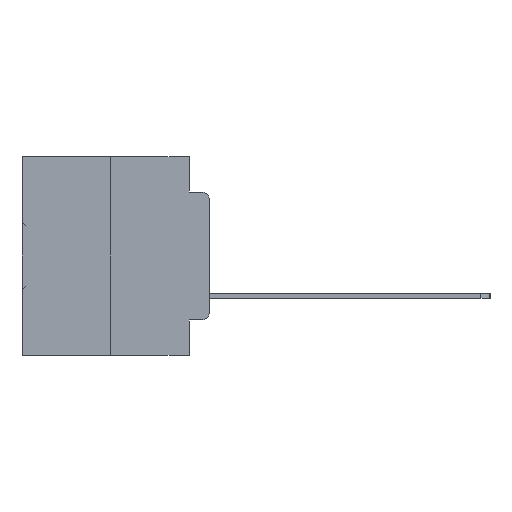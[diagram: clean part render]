
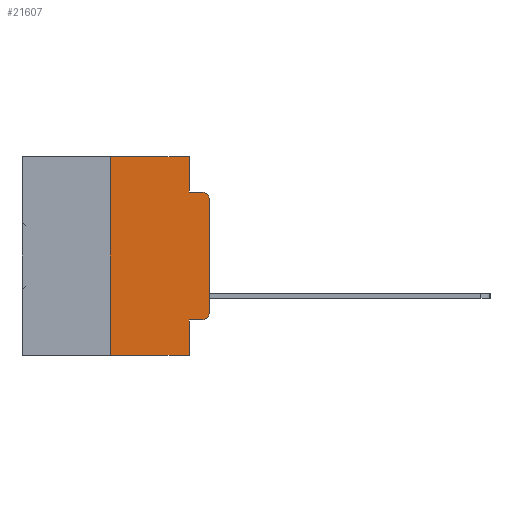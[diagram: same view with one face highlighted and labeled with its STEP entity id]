
A CAD part, left-side view. The second image highlights one B-rep face of the part: STEP entity #21607.
In plain terms, the highlighted planar face has unit normal (-1, 0, 0).
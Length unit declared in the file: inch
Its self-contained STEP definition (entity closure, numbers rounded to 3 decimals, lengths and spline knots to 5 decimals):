
#106 = CARTESIAN_POINT ( 'NONE',  ( 0., 0.051, -0.4115 ) ) ;
#803 = CARTESIAN_POINT ( 'NONE',  ( 0., 0.25, -0.5 ) ) ;
#1282 = DIRECTION ( 'NONE',  ( 0., 0., -1. ) ) ;
#1724 = LINE ( 'NONE', #18185, #30320 ) ;
#1936 = DIRECTION ( 'NONE',  ( 0., 0., 1. ) ) ;
#2275 = VERTEX_POINT ( 'NONE', #12704 ) ;
#3653 = LINE ( 'NONE', #31359, #10989 ) ;
#3901 = DIRECTION ( 'NONE',  ( 0., -1., 0. ) ) ;
#4256 = AXIS2_PLACEMENT_3D ( 'NONE', #33315, #17542, #1282 ) ;
#4645 = VECTOR ( 'NONE', #8822, 39.37008 ) ;
#4947 = CARTESIAN_POINT ( 'NONE',  ( 0., 0.02, -0.0885 ) ) ;
#5343 = EDGE_CURVE ( 'NONE', #2275, #32566, #19039, .T. ) ;
#6269 = LINE ( 'NONE', #21339, #19762 ) ;
#6331 = DIRECTION ( 'NONE',  ( -1., 0., 0. ) ) ;
#6492 = DIRECTION ( 'NONE',  ( 0., 0., -1. ) ) ;
#6609 = CARTESIAN_POINT ( 'NONE',  ( 0., 0., -0.1085 ) ) ;
#7224 = EDGE_CURVE ( 'NONE', #26252, #18542, #3653, .T. ) ;
#8822 = DIRECTION ( 'NONE',  ( 0., 0., -1. ) ) ;
#9346 = ORIENTED_EDGE ( 'NONE', *, *, #18053, .T. ) ;
#9942 = AXIS2_PLACEMENT_3D ( 'NONE', #22439, #6331, #22905 ) ;
#10749 = FACE_OUTER_BOUND ( 'NONE', #29321, .T. ) ;
#10989 = VECTOR ( 'NONE', #33819, 39.37008 ) ;
#12540 = CIRCLE ( 'NONE', #4256, 0.02 ) ;
#12704 = CARTESIAN_POINT ( 'NONE',  ( 0., 0.051, -0.4115 ) ) ;
#12747 = CIRCLE ( 'NONE', #9942, 0.02 ) ;
#13195 = ORIENTED_EDGE ( 'NONE', *, *, #25223, .T. ) ;
#13606 = VECTOR ( 'NONE', #6492, 39.37008 ) ;
#13950 = VECTOR ( 'NONE', #3901, 39.37008 ) ;
#14075 = DIRECTION ( 'NONE',  ( 1., 0., 0. ) ) ;
#14425 = ORIENTED_EDGE ( 'NONE', *, *, #5343, .F. ) ;
#14478 = CARTESIAN_POINT ( 'NONE',  ( 0., 0.051, -0.0885 ) ) ;
#14525 = EDGE_CURVE ( 'NONE', #18369, #19842, #34598, .T. ) ;
#14747 = LINE ( 'NONE', #30639, #13950 ) ;
#15618 = ORIENTED_EDGE ( 'NONE', *, *, #30724, .F. ) ;
#16273 = EDGE_CURVE ( 'NONE', #19842, #24676, #14747, .T. ) ;
#16492 = DIRECTION ( 'NONE',  ( 0., -1., 0. ) ) ;
#16880 = ORIENTED_EDGE ( 'NONE', *, *, #34581, .T. ) ;
#17285 = ORIENTED_EDGE ( 'NONE', *, *, #7224, .F. ) ;
#17542 = DIRECTION ( 'NONE',  ( -1., 0., 0. ) ) ;
#18053 = EDGE_CURVE ( 'NONE', #32202, #24676, #12747, .T. ) ;
#18185 = CARTESIAN_POINT ( 'NONE',  ( 0., 0., 0. ) ) ;
#18369 = VERTEX_POINT ( 'NONE', #29629 ) ;
#18542 = VERTEX_POINT ( 'NONE', #30295 ) ;
#18941 = ORIENTED_EDGE ( 'NONE', *, *, #20286, .T. ) ;
#19039 = LINE ( 'NONE', #22160, #4645 ) ;
#19762 = VECTOR ( 'NONE', #31948, 39.37008 ) ;
#19842 = VERTEX_POINT ( 'NONE', #14478 ) ;
#20095 = VERTEX_POINT ( 'NONE', #28839 ) ;
#20286 = EDGE_CURVE ( 'NONE', #26252, #32566, #31198, .T. ) ;
#21339 = CARTESIAN_POINT ( 'NONE',  ( 0., 0.473, 0. ) ) ;
#21607 = ADVANCED_FACE ( 'NONE', ( #10749 ), #24648, .F. ) ;
#22060 = VECTOR ( 'NONE', #27166, 39.37008 ) ;
#22160 = CARTESIAN_POINT ( 'NONE',  ( 0., 0.051, 0. ) ) ;
#22439 = CARTESIAN_POINT ( 'NONE',  ( 0., 0.02, -0.1085 ) ) ;
#22594 = CARTESIAN_POINT ( 'NONE',  ( 0., 0.051, 0. ) ) ;
#22874 = LINE ( 'NONE', #106, #22060 ) ;
#22905 = DIRECTION ( 'NONE',  ( 0., 0., -1. ) ) ;
#24215 = VECTOR ( 'NONE', #16492, 39.37008 ) ;
#24262 = VERTEX_POINT ( 'NONE', #24804 ) ;
#24648 = PLANE ( 'NONE',  #33973 ) ;
#24676 = VERTEX_POINT ( 'NONE', #4947 ) ;
#24804 = CARTESIAN_POINT ( 'NONE',  ( 0., 0., -0.3915 ) ) ;
#25223 = EDGE_CURVE ( 'NONE', #24262, #32202, #1724, .T. ) ;
#26252 = VERTEX_POINT ( 'NONE', #803 ) ;
#26450 = ORIENTED_EDGE ( 'NONE', *, *, #14525, .F. ) ;
#26484 = ORIENTED_EDGE ( 'NONE', *, *, #32853, .T. ) ;
#27166 = DIRECTION ( 'NONE',  ( 0., -1., 0. ) ) ;
#28839 = CARTESIAN_POINT ( 'NONE',  ( 0., 0.02, -0.4115 ) ) ;
#29321 = EDGE_LOOP ( 'NONE', ( #13195, #9346, #30135, #26450, #15618, #17285, #18941, #14425, #16880, #26484 ) ) ;
#29629 = CARTESIAN_POINT ( 'NONE',  ( 0., 0.051, 0. ) ) ;
#29936 = CARTESIAN_POINT ( 'NONE',  ( 0., 0.473, 0. ) ) ;
#30135 = ORIENTED_EDGE ( 'NONE', *, *, #16273, .F. ) ;
#30295 = CARTESIAN_POINT ( 'NONE',  ( 0., 0.25, 0. ) ) ;
#30320 = VECTOR ( 'NONE', #1936, 39.37008 ) ;
#30639 = CARTESIAN_POINT ( 'NONE',  ( 0., 0.051, -0.0885 ) ) ;
#30724 = EDGE_CURVE ( 'NONE', #18542, #18369, #6269, .T. ) ;
#31198 = LINE ( 'NONE', #32316, #24215 ) ;
#31359 = CARTESIAN_POINT ( 'NONE',  ( 0., 0.25, 0. ) ) ;
#31948 = DIRECTION ( 'NONE',  ( 0., -1., 0. ) ) ;
#32202 = VERTEX_POINT ( 'NONE', #6609 ) ;
#32316 = CARTESIAN_POINT ( 'NONE',  ( 0., 0.473, -0.5 ) ) ;
#32532 = DIRECTION ( 'NONE',  ( 0., 0., -1. ) ) ;
#32566 = VERTEX_POINT ( 'NONE', #34596 ) ;
#32853 = EDGE_CURVE ( 'NONE', #20095, #24262, #12540, .T. ) ;
#33315 = CARTESIAN_POINT ( 'NONE',  ( 0., 0.02, -0.3915 ) ) ;
#33819 = DIRECTION ( 'NONE',  ( 0., 0., 1. ) ) ;
#33973 = AXIS2_PLACEMENT_3D ( 'NONE', #29936, #14075, #32532 ) ;
#34581 = EDGE_CURVE ( 'NONE', #2275, #20095, #22874, .T. ) ;
#34596 = CARTESIAN_POINT ( 'NONE',  ( 0., 0.051, -0.5 ) ) ;
#34598 = LINE ( 'NONE', #22594, #13606 ) ;
